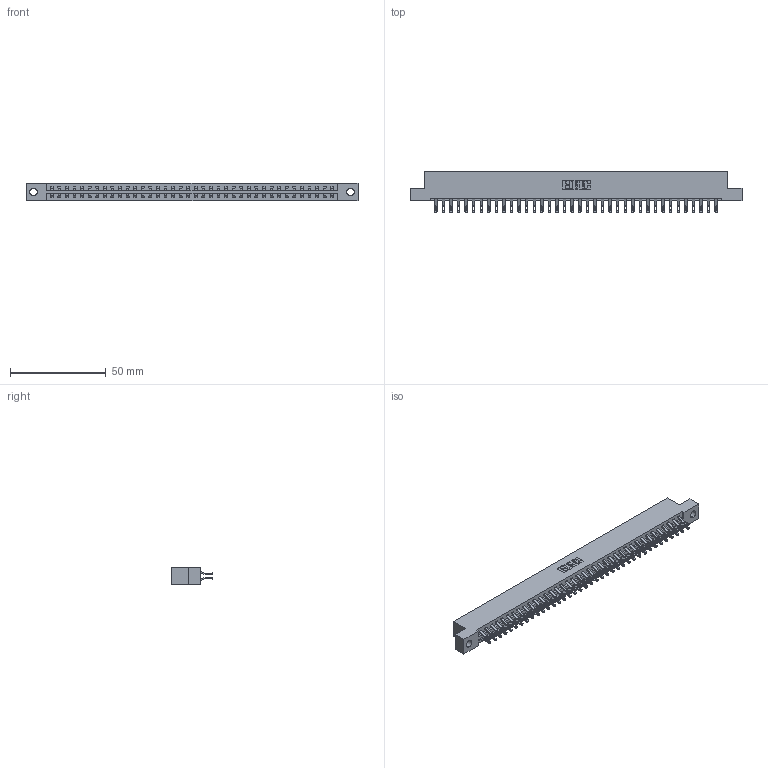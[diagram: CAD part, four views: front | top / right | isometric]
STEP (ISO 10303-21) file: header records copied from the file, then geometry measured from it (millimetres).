
FILE_DESCRIPTION (( 'STEP AP203' ), '1' );
FILE_NAME ('337-076-555-204.STEP', '2018-08-12T14:32:18', ( '' ), ( '' ), 'SwSTEP 2.0', 'SolidWorks 2016', '' );
FILE_SCHEMA (( 'CONFIG_CONTROL_DESIGN' ));
Length unit declared in the file: inch
Products named in the file (3): 337-076-555-204; 337 Part_Flush Mounting Lugs - 0.156 Dia-TH; 345-292-001_555 Tail
Assembly tree (77 placements, depth 2):
  337-076-555-204
    337 Part_Flush Mounting Lugs - 0.156 Dia-TH
    345-292-001_555 Tail  x76
Bounding box: 173.58 x 21.47 x 9.4 mm (x, y, z)
Volume: 18373 mm3; surface area: 21359.9 mm2
Topology: 77 solids, 77 shells, 4674 faces, 14675 edges, 9782 vertices
Faces by surface type: plane 2806, cylinder 1868
Entity records: 30309 total; most frequent: CARTESIAN_POINT 5144, ORIENTED_EDGE 5050, DIRECTION 4353, EDGE_CURVE 2525, LINE 2377, VECTOR 2377, VERTEX_POINT 1682, AXIS2_PLACEMENT_3D 988
